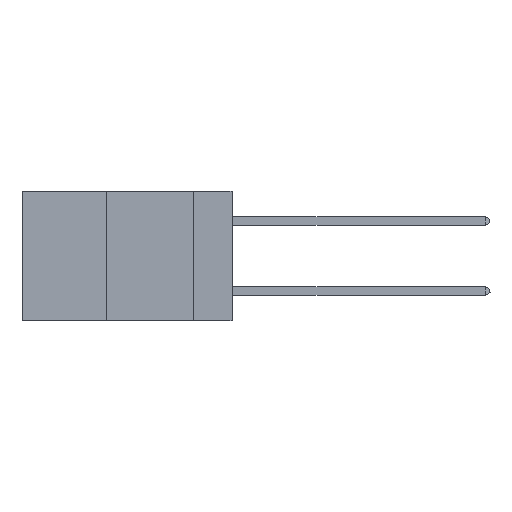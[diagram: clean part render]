
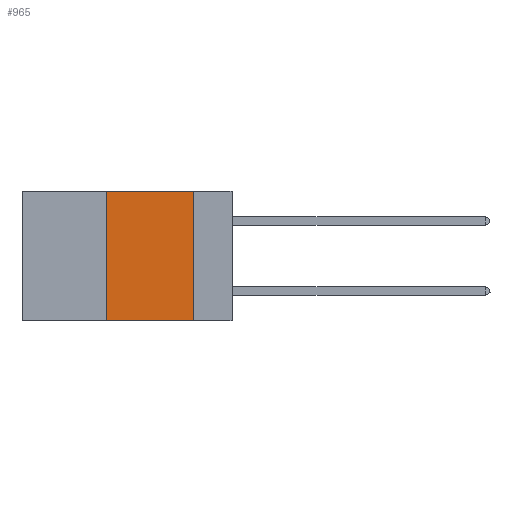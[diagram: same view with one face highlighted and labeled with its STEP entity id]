
A CAD part, left-side view. The second image highlights one B-rep face of the part: STEP entity #965.
In plain terms, the highlighted planar face has unit normal (-1, 0, 0).
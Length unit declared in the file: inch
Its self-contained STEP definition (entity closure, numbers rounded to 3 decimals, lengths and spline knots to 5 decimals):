
#530 = CARTESIAN_POINT ( 'NONE',  ( 0., 0.36, 0. ) ) ;
#721 = ORIENTED_EDGE ( 'NONE', *, *, #19908, .T. ) ;
#965 = ADVANCED_FACE ( 'NONE', ( #23052 ), #11920, .F. ) ;
#1212 = EDGE_CURVE ( 'NONE', #20366, #5657, #10531, .T. ) ;
#3194 = VECTOR ( 'NONE', #6200, 39.37008 ) ;
#3423 = CARTESIAN_POINT ( 'NONE',  ( 0., 0.11, 0. ) ) ;
#3551 = VERTEX_POINT ( 'NONE', #3423 ) ;
#4252 = DIRECTION ( 'NONE',  ( 1., 0., 0. ) ) ;
#4455 = ORIENTED_EDGE ( 'NONE', *, *, #4857, .F. ) ;
#4726 = ORIENTED_EDGE ( 'NONE', *, *, #15431, .F. ) ;
#4857 = EDGE_CURVE ( 'NONE', #5657, #3551, #25462, .T. ) ;
#5163 = VECTOR ( 'NONE', #16959, 39.37008 ) ;
#5187 = DIRECTION ( 'NONE',  ( 0., -1., 0. ) ) ;
#5266 = VERTEX_POINT ( 'NONE', #19291 ) ;
#5657 = VERTEX_POINT ( 'NONE', #530 ) ;
#5658 = AXIS2_PLACEMENT_3D ( 'NONE', #8212, #4252, #20282 ) ;
#6200 = DIRECTION ( 'NONE',  ( 0., -1., 0. ) ) ;
#8211 = CARTESIAN_POINT ( 'NONE',  ( 0., 0.6, 0. ) ) ;
#8212 = CARTESIAN_POINT ( 'NONE',  ( 0., 0.6, 0. ) ) ;
#9254 = CARTESIAN_POINT ( 'NONE',  ( 0., 0.36, -0.37 ) ) ;
#10122 = LINE ( 'NONE', #18070, #12358 ) ;
#10531 = LINE ( 'NONE', #21137, #5163 ) ;
#11338 = LINE ( 'NONE', #19271, #24768 ) ;
#11920 = PLANE ( 'NONE',  #5658 ) ;
#12149 = EDGE_LOOP ( 'NONE', ( #4726, #4455, #20191, #721 ) ) ;
#12358 = VECTOR ( 'NONE', #20152, 39.37008 ) ;
#15431 = EDGE_CURVE ( 'NONE', #3551, #5266, #10122, .T. ) ;
#16959 = DIRECTION ( 'NONE',  ( 0., 0., 1. ) ) ;
#18070 = CARTESIAN_POINT ( 'NONE',  ( 0., 0.11, 0. ) ) ;
#19271 = CARTESIAN_POINT ( 'NONE',  ( 0., 0.6, -0.37 ) ) ;
#19291 = CARTESIAN_POINT ( 'NONE',  ( 0., 0.11, -0.37 ) ) ;
#19908 = EDGE_CURVE ( 'NONE', #20366, #5266, #11338, .T. ) ;
#20152 = DIRECTION ( 'NONE',  ( 0., 0., -1. ) ) ;
#20191 = ORIENTED_EDGE ( 'NONE', *, *, #1212, .F. ) ;
#20282 = DIRECTION ( 'NONE',  ( 0., 0., -1. ) ) ;
#20366 = VERTEX_POINT ( 'NONE', #9254 ) ;
#21137 = CARTESIAN_POINT ( 'NONE',  ( 0., 0.36, 0. ) ) ;
#23052 = FACE_OUTER_BOUND ( 'NONE', #12149, .T. ) ;
#24768 = VECTOR ( 'NONE', #5187, 39.37008 ) ;
#25462 = LINE ( 'NONE', #8211, #3194 ) ;
